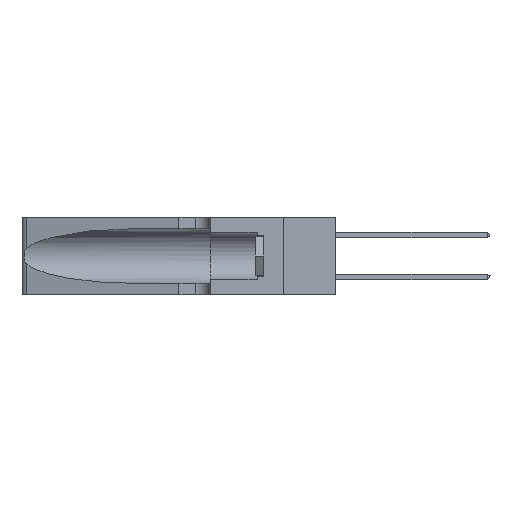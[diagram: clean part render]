
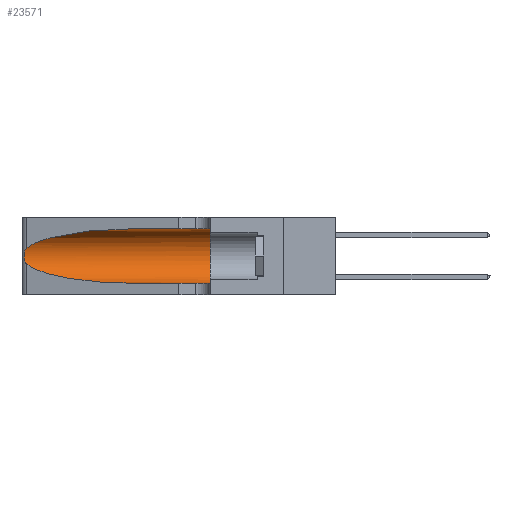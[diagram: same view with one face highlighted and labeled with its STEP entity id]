
A CAD part, left-side view. The second image highlights one B-rep face of the part: STEP entity #23571.
In plain terms, the highlighted cylindrical face has radius 3.308 mm (diameter 6.617 mm), a partial arc.
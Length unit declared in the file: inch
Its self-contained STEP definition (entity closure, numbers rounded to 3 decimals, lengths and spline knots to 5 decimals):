
#488 = DIRECTION ( 'NONE',  ( 0., -1., 0. ) ) ;
#1287 = CARTESIAN_POINT ( 'NONE',  ( 0.1305, 1.61858, 0.05475 ) ) ;
#1719 = CARTESIAN_POINT ( 'NONE',  ( 0.25487, 1.22718, 0.14631 ) ) ;
#2053 = LINE ( 'NONE', #1287, #7617 ) ;
#2271 = AXIS2_PLACEMENT_3D ( 'NONE', #6843, #6561, #22320 ) ;
#2437 = CARTESIAN_POINT ( 'NONE',  ( 0.1305, 0.72297, 0.31525 ) ) ;
#2473 = DIRECTION ( 'NONE',  ( 0., 1., 0. ) ) ;
#2831 = ORIENTED_EDGE ( 'NONE', *, *, #26664, .F. ) ;
#3331 = VERTEX_POINT ( 'NONE', #5160 ) ;
#3432 = CARTESIAN_POINT ( 'NONE',  ( 0.25487, 1.22718, 0.14631 ) ) ;
#3842 = CARTESIAN_POINT ( 'NONE',  ( 0.25789, 1.23486, 0.15765 ) ) ;
#3989 = EDGE_CURVE ( 'NONE', #3331, #27042, #7561, .T. ) ;
#4174 = VERTEX_POINT ( 'NONE', #3432 ) ;
#5160 = CARTESIAN_POINT ( 'NONE',  ( 0.1305, 0.35, 0.31525 ) ) ;
#5779 = CARTESIAN_POINT ( 'NONE',  ( 0.26018, 1.23835, 0.19895 ) ) ;
#5974 = CARTESIAN_POINT ( 'NONE',  ( 0.25487, 1.22718, 0.22369 ) ) ;
#6561 = DIRECTION ( 'NONE',  ( 0., -1., 0. ) ) ;
#6843 = CARTESIAN_POINT ( 'NONE',  ( 0.1305, 1.61858, 0.185 ) ) ;
#7561 = CIRCLE ( 'NONE', #8395, 0.13025 ) ;
#7617 = VECTOR ( 'NONE', #25640, 39.37008 ) ;
#7710 = B_SPLINE_CURVE_WITH_KNOTS ( 'NONE', 3,
 ( #5974, #8235, #10267, #14816, #14715, #5779, #18964, #23669, #19259, #21274, #3842, #8132, #19361, #1719 ),
 .UNSPECIFIED., .F., .F.,
 ( 4, 2, 2, 2, 2, 2, 4 ),
 ( 0., 0.00027, 0.00053, 0.00107, 0.0016, 0.00187, 0.00214 ),
 .UNSPECIFIED. ) ;
#7945 = CARTESIAN_POINT ( 'NONE',  ( 0.25487, 1.22718, 0.22369 ) ) ;
#8132 = CARTESIAN_POINT ( 'NONE',  ( 0.25639, 1.23186, 0.15144 ) ) ;
#8235 = CARTESIAN_POINT ( 'NONE',  ( 0.25555, 1.22994, 0.2215 ) ) ;
#8316 = CARTESIAN_POINT ( 'NONE',  ( 0.25487, 1.22718, 0.22369 ) ) ;
#8395 = AXIS2_PLACEMENT_3D ( 'NONE', #9180, #2473, #24797 ) ;
#8701 = LINE ( 'NONE', #13579, #26996 ) ;
#9180 = CARTESIAN_POINT ( 'NONE',  ( 0.1305, 0.35, 0.185 ) ) ;
#10167 = CARTESIAN_POINT ( 'NONE',  ( 0.18966, 0.96281, 0.31525 ) ) ;
#10267 = CARTESIAN_POINT ( 'NONE',  ( 0.25639, 1.23184, 0.21858 ) ) ;
#11423 = CYLINDRICAL_SURFACE ( 'NONE', #2271, 0.13025 ) ;
#11436 = VERTEX_POINT ( 'NONE', #2437 ) ;
#11495 = ORIENTED_EDGE ( 'NONE', *, *, #28278, .T. ) ;
#12305 = ORIENTED_EDGE ( 'NONE', *, *, #15364, .T. ) ;
#12732 = ORIENTED_EDGE ( 'NONE', *, *, #16160, .T. ) ;
#12883 = VERTEX_POINT ( 'NONE', #8316 ) ;
#13579 = CARTESIAN_POINT ( 'NONE',  ( 0.1305, 1.61858, 0.31525 ) ) ;
#14715 = CARTESIAN_POINT ( 'NONE',  ( 0.25854, 1.2359, 0.20912 ) ) ;
#14816 = CARTESIAN_POINT ( 'NONE',  ( 0.25787, 1.23484, 0.2124 ) ) ;
#14906 = CARTESIAN_POINT ( 'NONE',  ( 0.2373, 1.15595, 0.28018 ) ) ;
#15364 = EDGE_CURVE ( 'NONE', #21923, #27042, #2053, .T. ) ;
#15541 =( BOUNDED_CURVE ( )  B_SPLINE_CURVE ( 3, ( #27782, #27682, #19000, #21406 ),
 .UNSPECIFIED., .F., .F. ) 
 B_SPLINE_CURVE_WITH_KNOTS ( ( 4, 4 ),
 ( 3.44316, 4.71239 ),
 .UNSPECIFIED. ) 
 CURVE ( )  GEOMETRIC_REPRESENTATION_ITEM ( )  RATIONAL_B_SPLINE_CURVE ( ( 1., 0.87, 0.87, 1. ) ) 
 REPRESENTATION_ITEM ( '' )  );
#16160 = EDGE_CURVE ( 'NONE', #4174, #21923, #15541, .T. ) ;
#17306 = FACE_OUTER_BOUND ( 'NONE', #25960, .T. ) ;
#17336 = CARTESIAN_POINT ( 'NONE',  ( 0.1305, 0.35, 0.05475 ) ) ;
#18702 = ORIENTED_EDGE ( 'NONE', *, *, #3989, .F. ) ;
#18964 = CARTESIAN_POINT ( 'NONE',  ( 0.26075, 1.23896, 0.19203 ) ) ;
#19000 = CARTESIAN_POINT ( 'NONE',  ( 0.18966, 0.96281, 0.05475 ) ) ;
#19259 = CARTESIAN_POINT ( 'NONE',  ( 0.26017, 1.23833, 0.17102 ) ) ;
#19361 = CARTESIAN_POINT ( 'NONE',  ( 0.25555, 1.22993, 0.14849 ) ) ;
#21173 = CARTESIAN_POINT ( 'NONE',  ( 0.1305, 0.72297, 0.31525 ) ) ;
#21274 = CARTESIAN_POINT ( 'NONE',  ( 0.25856, 1.23593, 0.16098 ) ) ;
#21406 = CARTESIAN_POINT ( 'NONE',  ( 0.1305, 0.72297, 0.05475 ) ) ;
#21923 = VERTEX_POINT ( 'NONE', #25388 ) ;
#22320 = DIRECTION ( 'NONE',  ( 0., 0., -1. ) ) ;
#23571 = ADVANCED_FACE ( 'NONE', ( #17306 ), #11423, .F. ) ;
#23669 = CARTESIAN_POINT ( 'NONE',  ( 0.26075, 1.23896, 0.178 ) ) ;
#24797 = DIRECTION ( 'NONE',  ( 0., 0., 1. ) ) ;
#25205 = ORIENTED_EDGE ( 'NONE', *, *, #28343, .T. ) ;
#25388 = CARTESIAN_POINT ( 'NONE',  ( 0.1305, 0.72297, 0.05475 ) ) ;
#25640 = DIRECTION ( 'NONE',  ( 0., -1., 0. ) ) ;
#25760 =( BOUNDED_CURVE ( )  B_SPLINE_CURVE ( 3, ( #21173, #10167, #14906, #7945 ),
 .UNSPECIFIED., .F., .T. ) 
 B_SPLINE_CURVE_WITH_KNOTS ( ( 4, 4 ),
 ( 1.5708, 2.84003 ),
 .UNSPECIFIED. ) 
 CURVE ( )  GEOMETRIC_REPRESENTATION_ITEM ( )  RATIONAL_B_SPLINE_CURVE ( ( 1., 0.87, 0.87, 1. ) ) 
 REPRESENTATION_ITEM ( '' )  );
#25960 = EDGE_LOOP ( 'NONE', ( #11495, #25205, #12732, #12305, #18702, #2831 ) ) ;
#26664 = EDGE_CURVE ( 'NONE', #11436, #3331, #8701, .T. ) ;
#26996 = VECTOR ( 'NONE', #488, 39.37008 ) ;
#27042 = VERTEX_POINT ( 'NONE', #17336 ) ;
#27682 = CARTESIAN_POINT ( 'NONE',  ( 0.2373, 1.15595, 0.08982 ) ) ;
#27782 = CARTESIAN_POINT ( 'NONE',  ( 0.25487, 1.22718, 0.14631 ) ) ;
#28278 = EDGE_CURVE ( 'NONE', #11436, #12883, #25760, .T. ) ;
#28343 = EDGE_CURVE ( 'NONE', #12883, #4174, #7710, .T. ) ;
